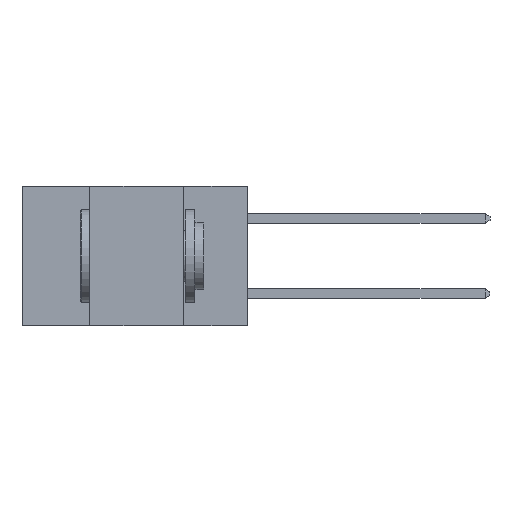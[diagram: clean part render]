
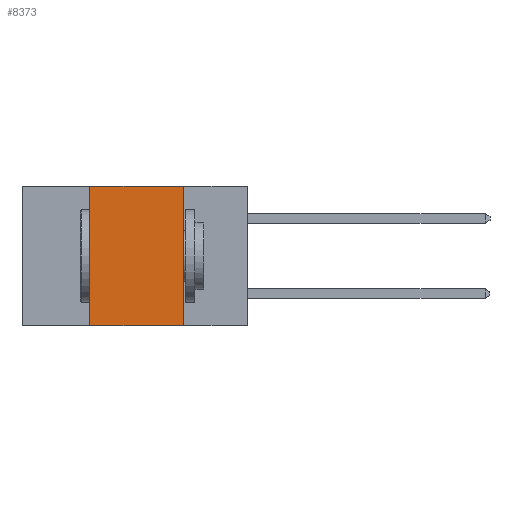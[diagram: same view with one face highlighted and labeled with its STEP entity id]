
A CAD part, left-side view. The second image highlights one B-rep face of the part: STEP entity #8373.
In plain terms, the highlighted planar face has unit normal (-1, 0, 0).
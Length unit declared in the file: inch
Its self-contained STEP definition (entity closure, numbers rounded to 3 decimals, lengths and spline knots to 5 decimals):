
#1986 = AXIS2_PLACEMENT_3D ( 'NONE', #10964, #10262, #10164 ) ;
#2012 = VECTOR ( 'NONE', #27985, 39.37008 ) ;
#2890 = CARTESIAN_POINT ( 'NONE',  ( 0., 0.17, -0.37 ) ) ;
#3340 = ORIENTED_EDGE ( 'NONE', *, *, #10217, .F. ) ;
#3558 = VECTOR ( 'NONE', #13643, 39.37008 ) ;
#4389 = FACE_OUTER_BOUND ( 'NONE', #6227, .T. ) ;
#4604 = DIRECTION ( 'NONE',  ( 0., -1., 0. ) ) ;
#5332 = VERTEX_POINT ( 'NONE', #8793 ) ;
#6227 = EDGE_LOOP ( 'NONE', ( #7109, #3340, #11905, #19713 ) ) ;
#7109 = ORIENTED_EDGE ( 'NONE', *, *, #14833, .F. ) ;
#7845 = LINE ( 'NONE', #8425, #2012 ) ;
#8373 = ADVANCED_FACE ( 'NONE', ( #4389 ), #10321, .F. ) ;
#8425 = CARTESIAN_POINT ( 'NONE',  ( 0., 0.17, 0. ) ) ;
#8739 = LINE ( 'NONE', #24202, #20292 ) ;
#8793 = CARTESIAN_POINT ( 'NONE',  ( 0., 0.42, 0. ) ) ;
#10164 = DIRECTION ( 'NONE',  ( 0., 0., -1. ) ) ;
#10217 = EDGE_CURVE ( 'NONE', #5332, #22562, #8739, .T. ) ;
#10262 = DIRECTION ( 'NONE',  ( 1., 0., 0. ) ) ;
#10321 = PLANE ( 'NONE',  #1986 ) ;
#10964 = CARTESIAN_POINT ( 'NONE',  ( 0., 0.6, 0. ) ) ;
#11075 = EDGE_CURVE ( 'NONE', #20456, #18981, #20911, .T. ) ;
#11408 = DIRECTION ( 'NONE',  ( 0., 0., 1. ) ) ;
#11489 = LINE ( 'NONE', #20045, #28117 ) ;
#11905 = ORIENTED_EDGE ( 'NONE', *, *, #27993, .F. ) ;
#13643 = DIRECTION ( 'NONE',  ( 0., -1., 0. ) ) ;
#14833 = EDGE_CURVE ( 'NONE', #22562, #18981, #7845, .T. ) ;
#16652 = CARTESIAN_POINT ( 'NONE',  ( 0., 0.17, 0. ) ) ;
#18981 = VERTEX_POINT ( 'NONE', #2890 ) ;
#19713 = ORIENTED_EDGE ( 'NONE', *, *, #11075, .T. ) ;
#20045 = CARTESIAN_POINT ( 'NONE',  ( 0., 0.42, 0. ) ) ;
#20292 = VECTOR ( 'NONE', #4604, 39.37008 ) ;
#20456 = VERTEX_POINT ( 'NONE', #22896 ) ;
#20911 = LINE ( 'NONE', #26637, #3558 ) ;
#22562 = VERTEX_POINT ( 'NONE', #16652 ) ;
#22896 = CARTESIAN_POINT ( 'NONE',  ( 0., 0.42, -0.37 ) ) ;
#24202 = CARTESIAN_POINT ( 'NONE',  ( 0., 0.6, 0. ) ) ;
#26637 = CARTESIAN_POINT ( 'NONE',  ( 0., 0.6, -0.37 ) ) ;
#27985 = DIRECTION ( 'NONE',  ( 0., 0., -1. ) ) ;
#27993 = EDGE_CURVE ( 'NONE', #20456, #5332, #11489, .T. ) ;
#28117 = VECTOR ( 'NONE', #11408, 39.37008 ) ;
